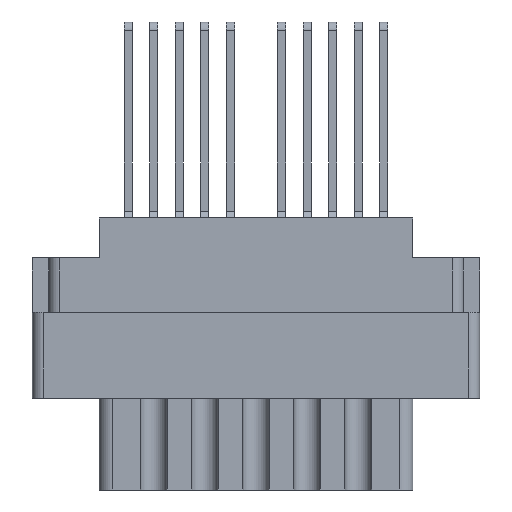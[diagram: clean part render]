
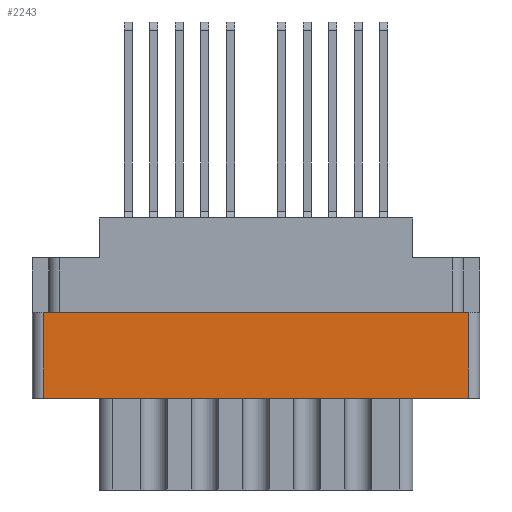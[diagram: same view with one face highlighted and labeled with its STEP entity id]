
A CAD part, front view. The second image highlights one B-rep face of the part: STEP entity #2243.
In plain terms, the highlighted planar face has unit normal (0, -1, 0).
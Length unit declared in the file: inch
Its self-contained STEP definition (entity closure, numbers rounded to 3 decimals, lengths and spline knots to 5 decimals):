
#66 = VECTOR ( 'NONE', #488, 39.37008 ) ;
#488 = DIRECTION ( 'NONE',  ( 0., 0., -1. ) ) ;
#533 = VERTEX_POINT ( 'NONE', #951 ) ;
#951 = CARTESIAN_POINT ( 'NONE',  ( -0.624, -0.343, -0.529 ) ) ;
#2243 = ADVANCED_FACE ( 'NONE', ( #26458 ), #18534, .T. ) ;
#2837 = LINE ( 'NONE', #3806, #3855 ) ;
#2849 = CARTESIAN_POINT ( 'NONE',  ( -0.624, -0.343, -0.798 ) ) ;
#3455 = DIRECTION ( 'NONE',  ( 0., -1., 0. ) ) ;
#3806 = CARTESIAN_POINT ( 'NONE',  ( 0., -0.343, -0.529 ) ) ;
#3855 = VECTOR ( 'NONE', #14776, 39.37008 ) ;
#4325 = CARTESIAN_POINT ( 'NONE',  ( 0., -0.343, -0.277 ) ) ;
#4751 = VERTEX_POINT ( 'NONE', #13311 ) ;
#5648 = EDGE_LOOP ( 'NONE', ( #14183, #8046, #6398, #17272 ) ) ;
#5672 = VECTOR ( 'NONE', #10199, 39.37008 ) ;
#6398 = ORIENTED_EDGE ( 'NONE', *, *, #24413, .F. ) ;
#8046 = ORIENTED_EDGE ( 'NONE', *, *, #8987, .T. ) ;
#8085 = EDGE_CURVE ( 'NONE', #16677, #24581, #16512, .T. ) ;
#8313 = AXIS2_PLACEMENT_3D ( 'NONE', #14331, #3455, #16527 ) ;
#8744 = LINE ( 'NONE', #21218, #5672 ) ;
#8850 = CARTESIAN_POINT ( 'NONE',  ( 0.624, -0.343, -0.277 ) ) ;
#8987 = EDGE_CURVE ( 'NONE', #16677, #533, #18511, .T. ) ;
#10199 = DIRECTION ( 'NONE',  ( 0., 0., 1. ) ) ;
#13311 = CARTESIAN_POINT ( 'NONE',  ( 0.624, -0.343, -0.529 ) ) ;
#14183 = ORIENTED_EDGE ( 'NONE', *, *, #8085, .F. ) ;
#14331 = CARTESIAN_POINT ( 'NONE',  ( -0.656, -0.343, -0.798 ) ) ;
#14344 = CARTESIAN_POINT ( 'NONE',  ( -0.624, -0.343, -0.277 ) ) ;
#14776 = DIRECTION ( 'NONE',  ( -1., 0., 0. ) ) ;
#16512 = LINE ( 'NONE', #4325, #27136 ) ;
#16527 = DIRECTION ( 'NONE',  ( 0., 0., -1. ) ) ;
#16677 = VERTEX_POINT ( 'NONE', #14344 ) ;
#17272 = ORIENTED_EDGE ( 'NONE', *, *, #21416, .T. ) ;
#18511 = LINE ( 'NONE', #2849, #66 ) ;
#18534 = PLANE ( 'NONE',  #8313 ) ;
#21218 = CARTESIAN_POINT ( 'NONE',  ( 0.624, -0.343, -0.798 ) ) ;
#21416 = EDGE_CURVE ( 'NONE', #4751, #24581, #8744, .T. ) ;
#21552 = DIRECTION ( 'NONE',  ( 1., 0., 0. ) ) ;
#24413 = EDGE_CURVE ( 'NONE', #4751, #533, #2837, .T. ) ;
#24581 = VERTEX_POINT ( 'NONE', #8850 ) ;
#26458 = FACE_OUTER_BOUND ( 'NONE', #5648, .T. ) ;
#27136 = VECTOR ( 'NONE', #21552, 39.37008 ) ;
